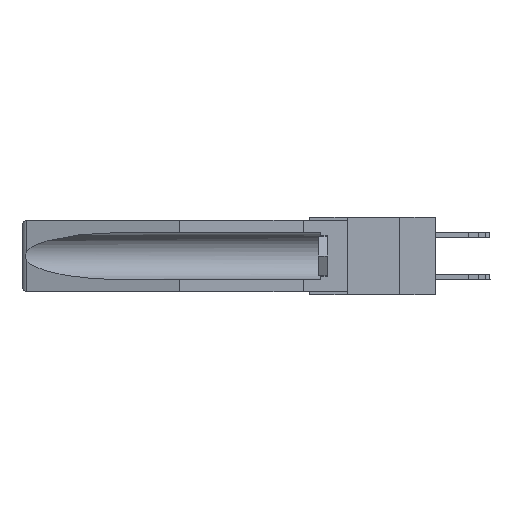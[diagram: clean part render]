
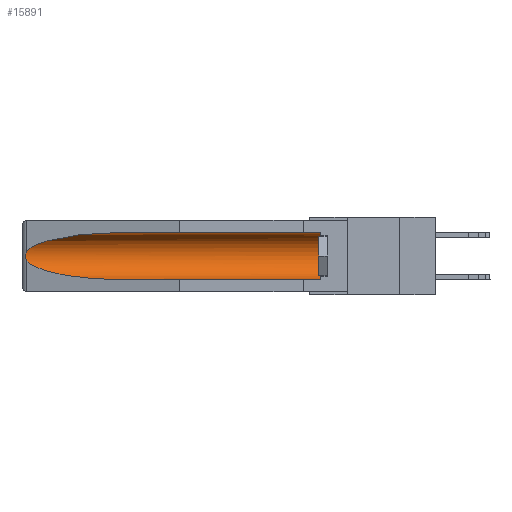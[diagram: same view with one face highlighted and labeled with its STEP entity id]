
A CAD part, left-side view. The second image highlights one B-rep face of the part: STEP entity #15891.
In plain terms, the highlighted cylindrical face has radius 2.857 mm (diameter 5.715 mm), a partial arc.
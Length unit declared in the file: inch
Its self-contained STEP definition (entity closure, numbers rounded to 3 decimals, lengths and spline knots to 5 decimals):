
#289 = VECTOR ( 'NONE', #15747, 39.37008 ) ;
#620 = DIRECTION ( 'NONE',  ( 0., 0., 1. ) ) ;
#669 = CARTESIAN_POINT ( 'NONE',  ( 0.2673, 1.53269, -0.17917 ) ) ;
#925 = CIRCLE ( 'NONE', #5936, 0.1125 ) ;
#1482 = CARTESIAN_POINT ( 'NONE',  ( 0.25451, 1.48313, -0.09465 ) ) ;
#1599 = CARTESIAN_POINT ( 'NONE',  ( 0.26537, 1.52718, -0.14972 ) ) ;
#2418 = CARTESIAN_POINT ( 'NONE',  ( 0.21114, 1.30732, -0.059 ) ) ;
#2495 = CARTESIAN_POINT ( 'NONE',  ( 0.26654, 1.53092, -0.15636 ) ) ;
#2642 = CARTESIAN_POINT ( 'NONE',  ( 0.2673, 1.5327, -0.16383 ) ) ;
#2697 = EDGE_CURVE ( 'NONE', #3459, #16885, #21144, .T. ) ;
#2950 = CARTESIAN_POINT ( 'NONE',  ( 0.155, 0.126, -0.059 ) ) ;
#3059 = DIRECTION ( 'NONE',  ( 0., 0., 1. ) ) ;
#3431 = CARTESIAN_POINT ( 'NONE',  ( 0.155, 1.07973, -0.059 ) ) ;
#3459 = VERTEX_POINT ( 'NONE', #8292 ) ;
#3484 = CARTESIAN_POINT ( 'NONE',  ( 0.25451, 1.48313, -0.24835 ) ) ;
#4447 = CARTESIAN_POINT ( 'NONE',  ( 0.26655, 1.53094, -0.18657 ) ) ;
#5105 = ORIENTED_EDGE ( 'NONE', *, *, #8590, .T. ) ;
#5364 = VERTEX_POINT ( 'NONE', #2950 ) ;
#5584 = CYLINDRICAL_SURFACE ( 'NONE', #10527, 0.1125 ) ;
#5936 = AXIS2_PLACEMENT_3D ( 'NONE', #8221, #10149, #3059 ) ;
#6991 = DIRECTION ( 'NONE',  ( 0., 1., 0. ) ) ;
#7012 = CARTESIAN_POINT ( 'NONE',  ( 0.155, 1.07973, -0.284 ) ) ;
#7486 = VERTEX_POINT ( 'NONE', #10419 ) ;
#7764 = DIRECTION ( 'NONE',  ( 0., 1., 0. ) ) ;
#8139 = VERTEX_POINT ( 'NONE', #13174 ) ;
#8221 = CARTESIAN_POINT ( 'NONE',  ( 0.155, 0.126, -0.1715 ) ) ;
#8292 = CARTESIAN_POINT ( 'NONE',  ( 0.155, 0.126, -0.284 ) ) ;
#8590 = EDGE_CURVE ( 'NONE', #7486, #16885, #22282, .T. ) ;
#10149 = DIRECTION ( 'NONE',  ( 0., -1., 0. ) ) ;
#10352 = ORIENTED_EDGE ( 'NONE', *, *, #16348, .T. ) ;
#10419 = CARTESIAN_POINT ( 'NONE',  ( 0.26537, 1.52718, -0.19328 ) ) ;
#10527 = AXIS2_PLACEMENT_3D ( 'NONE', #16824, #7764, #620 ) ;
#10640 = CARTESIAN_POINT ( 'NONE',  ( 0.155, -0.30754, -0.284 ) ) ;
#13174 = CARTESIAN_POINT ( 'NONE',  ( 0.26537, 1.52718, -0.14972 ) ) ;
#13812 = EDGE_CURVE ( 'NONE', #5364, #16137, #14707, .T. ) ;
#14308 = CARTESIAN_POINT ( 'NONE',  ( 0.21114, 1.30732, -0.284 ) ) ;
#14337 = ORIENTED_EDGE ( 'NONE', *, *, #20998, .T. ) ;
#14614 = VECTOR ( 'NONE', #6991, 39.37008 ) ;
#14707 = LINE ( 'NONE', #21014, #289 ) ;
#15071 = ORIENTED_EDGE ( 'NONE', *, *, #13812, .T. ) ;
#15374 = CARTESIAN_POINT ( 'NONE',  ( 0.2675, 1.53308, -0.17534 ) ) ;
#15747 = DIRECTION ( 'NONE',  ( 0., 1., 0. ) ) ;
#15891 = ADVANCED_FACE ( 'NONE', ( #17189 ), #5584, .F. ) ;
#16137 = VERTEX_POINT ( 'NONE', #3431 ) ;
#16348 = EDGE_CURVE ( 'NONE', #8139, #7486, #21533, .T. ) ;
#16824 = CARTESIAN_POINT ( 'NONE',  ( 0.155, -0.30754, -0.1715 ) ) ;
#16872 = CARTESIAN_POINT ( 'NONE',  ( 0.26597, 1.5296, -0.19026 ) ) ;
#16885 = VERTEX_POINT ( 'NONE', #20938 ) ;
#17027 = CARTESIAN_POINT ( 'NONE',  ( 0.26597, 1.52961, -0.15275 ) ) ;
#17189 = FACE_OUTER_BOUND ( 'NONE', #20426, .T. ) ;
#17515 = CARTESIAN_POINT ( 'NONE',  ( 0.155, 1.07973, -0.059 ) ) ;
#18676 =( BOUNDED_CURVE ( )  B_SPLINE_CURVE ( 3, ( #17515, #2418, #1482, #1599 ),
 .UNSPECIFIED., .F., .F. ) 
 B_SPLINE_CURVE_WITH_KNOTS ( ( 4, 4 ),
 ( 4.71239, 6.08839 ),
 .UNSPECIFIED. ) 
 CURVE ( )  GEOMETRIC_REPRESENTATION_ITEM ( )  RATIONAL_B_SPLINE_CURVE ( ( 1., 0.848, 0.848, 1. ) ) 
 REPRESENTATION_ITEM ( '' )  );
#18703 = CARTESIAN_POINT ( 'NONE',  ( 0.26537, 1.52718, -0.19328 ) ) ;
#18921 = CARTESIAN_POINT ( 'NONE',  ( 0.2675, 1.53308, -0.16763 ) ) ;
#20426 = EDGE_LOOP ( 'NONE', ( #14337, #10352, #5105, #22999, #22227, #15071 ) ) ;
#20655 = CARTESIAN_POINT ( 'NONE',  ( 0.26537, 1.52718, -0.14972 ) ) ;
#20938 = CARTESIAN_POINT ( 'NONE',  ( 0.155, 1.07973, -0.284 ) ) ;
#20998 = EDGE_CURVE ( 'NONE', #16137, #8139, #18676, .T. ) ;
#21014 = CARTESIAN_POINT ( 'NONE',  ( 0.155, -0.30754, -0.059 ) ) ;
#21144 = LINE ( 'NONE', #10640, #14614 ) ;
#21533 = B_SPLINE_CURVE_WITH_KNOTS ( 'NONE', 3,
 ( #20655, #17027, #2495, #2642, #18921, #15374, #669, #4447, #16872, #18703 ),
 .UNSPECIFIED., .F., .F.,
 ( 4, 2, 2, 2, 4 ),
 ( 0., 0.00029, 0.00058, 0.00087, 0.00117 ),
 .UNSPECIFIED. ) ;
#21863 = CARTESIAN_POINT ( 'NONE',  ( 0.26537, 1.52718, -0.19328 ) ) ;
#22227 = ORIENTED_EDGE ( 'NONE', *, *, #22389, .T. ) ;
#22282 =( BOUNDED_CURVE ( )  B_SPLINE_CURVE ( 3, ( #21863, #3484, #14308, #7012 ),
 .UNSPECIFIED., .F., .F. ) 
 B_SPLINE_CURVE_WITH_KNOTS ( ( 4, 4 ),
 ( 0.1948, 1.5708 ),
 .UNSPECIFIED. ) 
 CURVE ( )  GEOMETRIC_REPRESENTATION_ITEM ( )  RATIONAL_B_SPLINE_CURVE ( ( 1., 0.848, 0.848, 1. ) ) 
 REPRESENTATION_ITEM ( '' )  );
#22389 = EDGE_CURVE ( 'NONE', #3459, #5364, #925, .T. ) ;
#22999 = ORIENTED_EDGE ( 'NONE', *, *, #2697, .F. ) ;
